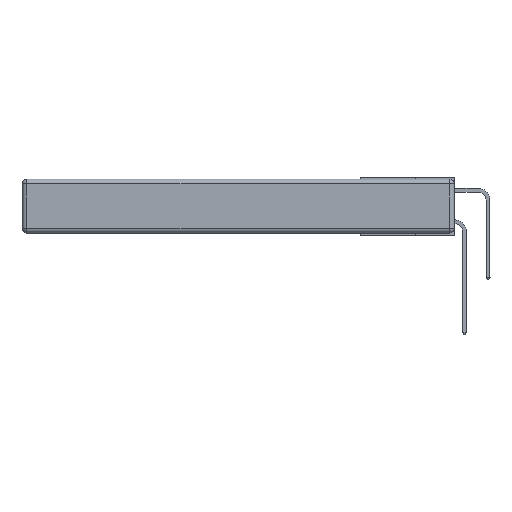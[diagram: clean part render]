
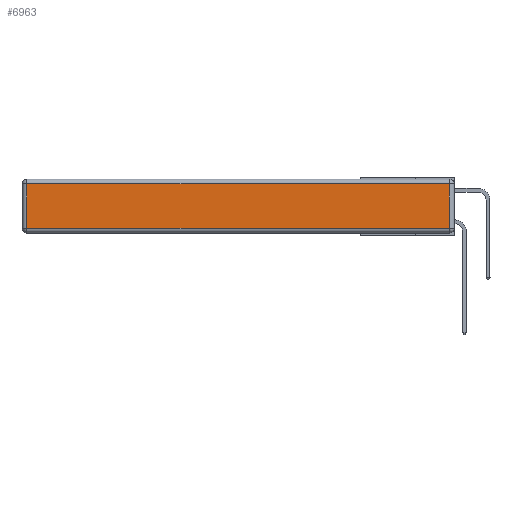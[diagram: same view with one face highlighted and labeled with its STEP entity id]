
A CAD part, left-side view. The second image highlights one B-rep face of the part: STEP entity #6963.
In plain terms, the highlighted planar face has unit normal (-1, 0, 0).
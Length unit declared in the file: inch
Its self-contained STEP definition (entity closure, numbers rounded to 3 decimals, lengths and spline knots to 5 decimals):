
#48 = VECTOR ( 'NONE', #686, 39.37008 ) ;
#193 = VECTOR ( 'NONE', #8081, 39.37008 ) ;
#219 = CARTESIAN_POINT ( 'NONE',  ( 0., 2.72, -0.343 ) ) ;
#623 = DIRECTION ( 'NONE',  ( 0., 0., 1. ) ) ;
#627 = CARTESIAN_POINT ( 'NONE',  ( 0., 2.75, -0.03 ) ) ;
#680 = PLANE ( 'NONE',  #7486 ) ;
#686 = DIRECTION ( 'NONE',  ( 0., 1., 0. ) ) ;
#1802 = DIRECTION ( 'NONE',  ( -1., 0., 0. ) ) ;
#2487 = CARTESIAN_POINT ( 'NONE',  ( 0., 0.03, -0.313 ) ) ;
#2562 = ORIENTED_EDGE ( 'NONE', *, *, #5775, .T. ) ;
#3525 = VECTOR ( 'NONE', #5815, 39.37008 ) ;
#3874 = CARTESIAN_POINT ( 'NONE',  ( 0., 0., -0.343 ) ) ;
#3945 = EDGE_LOOP ( 'NONE', ( #2562, #5744, #9298, #5672 ) ) ;
#5185 = EDGE_CURVE ( 'NONE', #13514, #12121, #8477, .T. ) ;
#5513 = EDGE_CURVE ( 'NONE', #7096, #13514, #11244, .T. ) ;
#5672 = ORIENTED_EDGE ( 'NONE', *, *, #5185, .T. ) ;
#5744 = ORIENTED_EDGE ( 'NONE', *, *, #8916, .T. ) ;
#5775 = EDGE_CURVE ( 'NONE', #12121, #9901, #8991, .T. ) ;
#5815 = DIRECTION ( 'NONE',  ( 0., 0., -1. ) ) ;
#6142 = LINE ( 'NONE', #6945, #193 ) ;
#6945 = CARTESIAN_POINT ( 'NONE',  ( 0., 0.03, -0.343 ) ) ;
#6963 = ADVANCED_FACE ( 'NONE', ( #13150 ), #680, .T. ) ;
#7096 = VERTEX_POINT ( 'NONE', #13138 ) ;
#7486 = AXIS2_PLACEMENT_3D ( 'NONE', #3874, #1802, #623 ) ;
#8081 = DIRECTION ( 'NONE',  ( 0., 0., 1. ) ) ;
#8099 = DIRECTION ( 'NONE',  ( 0., -1., 0. ) ) ;
#8477 = LINE ( 'NONE', #219, #3525 ) ;
#8916 = EDGE_CURVE ( 'NONE', #9901, #7096, #6142, .T. ) ;
#8991 = LINE ( 'NONE', #13726, #11603 ) ;
#9298 = ORIENTED_EDGE ( 'NONE', *, *, #5513, .T. ) ;
#9625 = CARTESIAN_POINT ( 'NONE',  ( 0., 2.72, -0.03 ) ) ;
#9901 = VERTEX_POINT ( 'NONE', #2487 ) ;
#11244 = LINE ( 'NONE', #627, #48 ) ;
#11603 = VECTOR ( 'NONE', #8099, 39.37008 ) ;
#12121 = VERTEX_POINT ( 'NONE', #13050 ) ;
#13050 = CARTESIAN_POINT ( 'NONE',  ( 0., 2.72, -0.313 ) ) ;
#13138 = CARTESIAN_POINT ( 'NONE',  ( 0., 0.03, -0.03 ) ) ;
#13150 = FACE_OUTER_BOUND ( 'NONE', #3945, .T. ) ;
#13514 = VERTEX_POINT ( 'NONE', #9625 ) ;
#13726 = CARTESIAN_POINT ( 'NONE',  ( 0., 0., -0.313 ) ) ;
